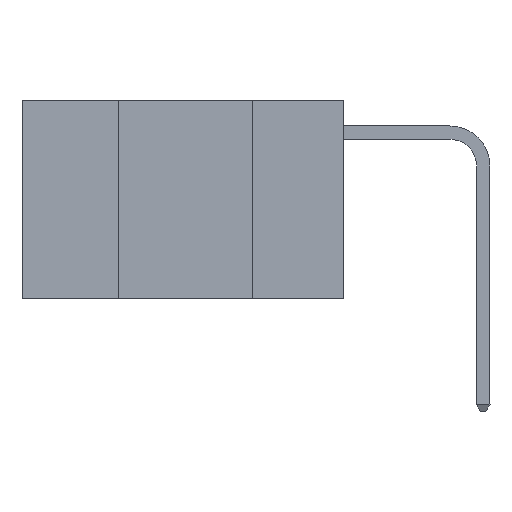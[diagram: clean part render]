
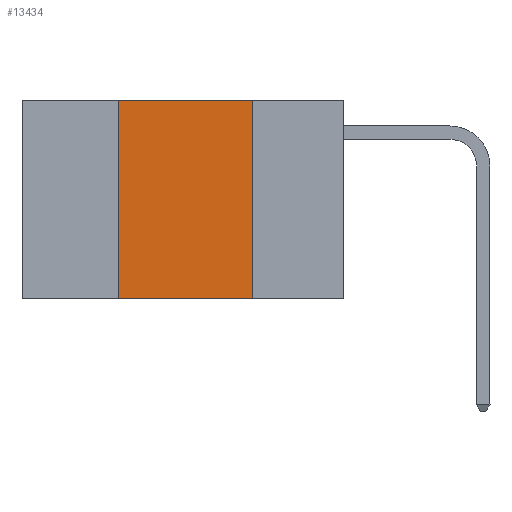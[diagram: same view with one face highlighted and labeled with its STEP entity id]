
A CAD part, left-side view. The second image highlights one B-rep face of the part: STEP entity #13434.
In plain terms, the highlighted planar face has unit normal (-1, 0, 0).
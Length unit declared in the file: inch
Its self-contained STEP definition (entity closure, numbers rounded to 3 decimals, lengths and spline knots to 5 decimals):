
#768 = CARTESIAN_POINT ( 'NONE',  ( 0., 0.17, -0.37 ) ) ;
#2289 = ORIENTED_EDGE ( 'NONE', *, *, #5383, .F. ) ;
#3295 = DIRECTION ( 'NONE',  ( 0., -1., 0. ) ) ;
#3508 = DIRECTION ( 'NONE',  ( 0., -1., 0. ) ) ;
#4853 = DIRECTION ( 'NONE',  ( 0., 0., -1. ) ) ;
#4945 = LINE ( 'NONE', #14683, #9112 ) ;
#4951 = DIRECTION ( 'NONE',  ( 0., 0., -1. ) ) ;
#5383 = EDGE_CURVE ( 'NONE', #11875, #9738, #4945, .T. ) ;
#6114 = CARTESIAN_POINT ( 'NONE',  ( 0., 0.42, 0. ) ) ;
#6342 = DIRECTION ( 'NONE',  ( 1., 0., 0. ) ) ;
#9012 = VECTOR ( 'NONE', #3508, 39.37008 ) ;
#9047 = ORIENTED_EDGE ( 'NONE', *, *, #12012, .T. ) ;
#9112 = VECTOR ( 'NONE', #4853, 39.37008 ) ;
#9435 = ORIENTED_EDGE ( 'NONE', *, *, #16033, .F. ) ;
#9738 = VERTEX_POINT ( 'NONE', #768 ) ;
#9828 = VECTOR ( 'NONE', #3295, 39.37008 ) ;
#9930 = EDGE_CURVE ( 'NONE', #10477, #15689, #10152, .T. ) ;
#10152 = LINE ( 'NONE', #6114, #15929 ) ;
#10477 = VERTEX_POINT ( 'NONE', #14694 ) ;
#10635 = PLANE ( 'NONE',  #11024 ) ;
#11024 = AXIS2_PLACEMENT_3D ( 'NONE', #14510, #6342, #4951 ) ;
#11848 = LINE ( 'NONE', #16097, #9012 ) ;
#11875 = VERTEX_POINT ( 'NONE', #16185 ) ;
#12012 = EDGE_CURVE ( 'NONE', #10477, #9738, #17384, .T. ) ;
#13290 = FACE_OUTER_BOUND ( 'NONE', #16206, .T. ) ;
#13397 = ORIENTED_EDGE ( 'NONE', *, *, #9930, .F. ) ;
#13434 = ADVANCED_FACE ( 'NONE', ( #13290 ), #10635, .F. ) ;
#13718 = CARTESIAN_POINT ( 'NONE',  ( 0., 0.42, 0. ) ) ;
#14509 = CARTESIAN_POINT ( 'NONE',  ( 0., 0.6, -0.37 ) ) ;
#14510 = CARTESIAN_POINT ( 'NONE',  ( 0., 0.6, 0. ) ) ;
#14683 = CARTESIAN_POINT ( 'NONE',  ( 0., 0.17, 0. ) ) ;
#14694 = CARTESIAN_POINT ( 'NONE',  ( 0., 0.42, -0.37 ) ) ;
#15689 = VERTEX_POINT ( 'NONE', #13718 ) ;
#15929 = VECTOR ( 'NONE', #16026, 39.37008 ) ;
#16026 = DIRECTION ( 'NONE',  ( 0., 0., 1. ) ) ;
#16033 = EDGE_CURVE ( 'NONE', #15689, #11875, #11848, .T. ) ;
#16097 = CARTESIAN_POINT ( 'NONE',  ( 0., 0.6, 0. ) ) ;
#16185 = CARTESIAN_POINT ( 'NONE',  ( 0., 0.17, 0. ) ) ;
#16206 = EDGE_LOOP ( 'NONE', ( #2289, #9435, #13397, #9047 ) ) ;
#17384 = LINE ( 'NONE', #14509, #9828 ) ;
